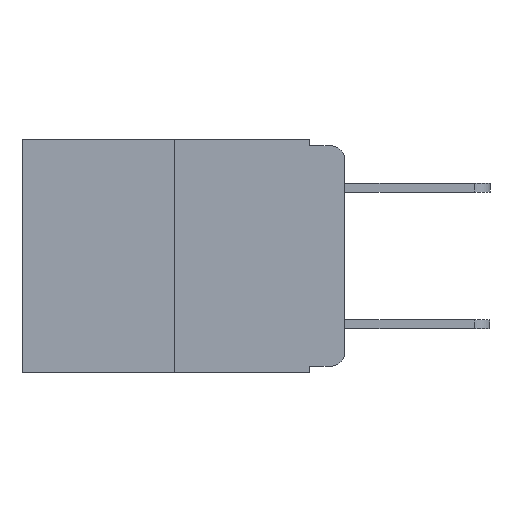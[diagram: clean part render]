
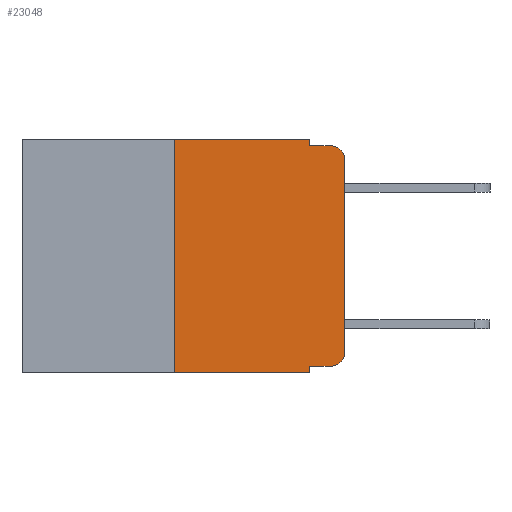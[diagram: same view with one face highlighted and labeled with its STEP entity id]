
A CAD part, left-side view. The second image highlights one B-rep face of the part: STEP entity #23048.
In plain terms, the highlighted planar face has unit normal (-1, 0, 0).
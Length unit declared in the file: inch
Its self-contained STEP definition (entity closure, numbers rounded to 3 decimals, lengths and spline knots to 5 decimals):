
#221 = CARTESIAN_POINT ( 'NONE',  ( 0., 0.02, -0.313 ) ) ;
#282 = CARTESIAN_POINT ( 'NONE',  ( 0., 0.051, -0.01 ) ) ;
#1136 = DIRECTION ( 'NONE',  ( 0., -1., 0. ) ) ;
#1621 = DIRECTION ( 'NONE',  ( 0., 0., -1. ) ) ;
#1648 = VECTOR ( 'NONE', #16089, 39.37008 ) ;
#2386 = DIRECTION ( 'NONE',  ( 0., 0., -1. ) ) ;
#2423 = ORIENTED_EDGE ( 'NONE', *, *, #12696, .T. ) ;
#2565 = LINE ( 'NONE', #9049, #16237 ) ;
#3537 = LINE ( 'NONE', #24974, #13744 ) ;
#3592 = CIRCLE ( 'NONE', #25073, 0.02 ) ;
#4366 = VERTEX_POINT ( 'NONE', #23826 ) ;
#4707 = VERTEX_POINT ( 'NONE', #10649 ) ;
#5667 = LINE ( 'NONE', #11386, #20867 ) ;
#5887 = ORIENTED_EDGE ( 'NONE', *, *, #19730, .T. ) ;
#6065 = CARTESIAN_POINT ( 'NONE',  ( 0., 0.051, 0. ) ) ;
#6078 = EDGE_CURVE ( 'NONE', #4366, #4707, #7816, .T. ) ;
#6690 = ORIENTED_EDGE ( 'NONE', *, *, #21004, .T. ) ;
#6816 = CARTESIAN_POINT ( 'NONE',  ( 0., 0.25, -0.343 ) ) ;
#7063 = DIRECTION ( 'NONE',  ( 0., -1., 0. ) ) ;
#7084 = CARTESIAN_POINT ( 'NONE',  ( 0., 0., -0.03 ) ) ;
#7166 = VECTOR ( 'NONE', #18612, 39.37008 ) ;
#7433 = DIRECTION ( 'NONE',  ( 0., -1., 0. ) ) ;
#7816 = LINE ( 'NONE', #282, #7166 ) ;
#8288 = ORIENTED_EDGE ( 'NONE', *, *, #24489, .T. ) ;
#9049 = CARTESIAN_POINT ( 'NONE',  ( 0., 0.473, -0.343 ) ) ;
#9240 = ORIENTED_EDGE ( 'NONE', *, *, #9906, .F. ) ;
#9301 = ORIENTED_EDGE ( 'NONE', *, *, #25091, .T. ) ;
#9702 = EDGE_CURVE ( 'NONE', #19237, #4366, #18660, .T. ) ;
#9906 = EDGE_CURVE ( 'NONE', #10057, #19237, #3537, .T. ) ;
#10057 = VERTEX_POINT ( 'NONE', #13990 ) ;
#10649 = CARTESIAN_POINT ( 'NONE',  ( 0., 0.02, -0.01 ) ) ;
#10796 = LINE ( 'NONE', #11802, #20591 ) ;
#10855 = CARTESIAN_POINT ( 'NONE',  ( 0., 0.051, 0. ) ) ;
#10887 = VERTEX_POINT ( 'NONE', #7084 ) ;
#10892 = DIRECTION ( 'NONE',  ( 1., 0., 0. ) ) ;
#11386 = CARTESIAN_POINT ( 'NONE',  ( 0., 0.051, -0.333 ) ) ;
#11802 = CARTESIAN_POINT ( 'NONE',  ( 0., 0.25, 0. ) ) ;
#12675 = ORIENTED_EDGE ( 'NONE', *, *, #6078, .F. ) ;
#12696 = EDGE_CURVE ( 'NONE', #20695, #13056, #5667, .T. ) ;
#13056 = VERTEX_POINT ( 'NONE', #14496 ) ;
#13441 = ORIENTED_EDGE ( 'NONE', *, *, #9702, .F. ) ;
#13744 = VECTOR ( 'NONE', #1136, 39.37008 ) ;
#13931 = DIRECTION ( 'NONE',  ( -1., 0., 0. ) ) ;
#13990 = CARTESIAN_POINT ( 'NONE',  ( 0., 0.25, 0. ) ) ;
#14068 = VECTOR ( 'NONE', #24414, 39.37008 ) ;
#14496 = CARTESIAN_POINT ( 'NONE',  ( 0., 0.02, -0.333 ) ) ;
#14610 = DIRECTION ( 'NONE',  ( -1., 0., 0. ) ) ;
#15234 = CARTESIAN_POINT ( 'NONE',  ( 0., 0., -0.313 ) ) ;
#15466 = AXIS2_PLACEMENT_3D ( 'NONE', #25412, #13931, #1621 ) ;
#15663 = FACE_OUTER_BOUND ( 'NONE', #25450, .T. ) ;
#15791 = LINE ( 'NONE', #20997, #24137 ) ;
#16089 = DIRECTION ( 'NONE',  ( 0., 0., -1. ) ) ;
#16237 = VECTOR ( 'NONE', #7063, 39.37008 ) ;
#16926 = CARTESIAN_POINT ( 'NONE',  ( 0., 0.051, 0. ) ) ;
#17564 = CARTESIAN_POINT ( 'NONE',  ( 0., 0.051, -0.333 ) ) ;
#18462 = LINE ( 'NONE', #6065, #1648 ) ;
#18554 = CARTESIAN_POINT ( 'NONE',  ( 0., 0.051, -0.343 ) ) ;
#18612 = DIRECTION ( 'NONE',  ( 0., -1., 0. ) ) ;
#18660 = LINE ( 'NONE', #10855, #14068 ) ;
#19237 = VERTEX_POINT ( 'NONE', #16926 ) ;
#19533 = VERTEX_POINT ( 'NONE', #15234 ) ;
#19730 = EDGE_CURVE ( 'NONE', #10887, #4707, #20257, .T. ) ;
#19788 = EDGE_CURVE ( 'NONE', #20695, #21026, #18462, .T. ) ;
#20257 = CIRCLE ( 'NONE', #15466, 0.02 ) ;
#20591 = VECTOR ( 'NONE', #23388, 39.37008 ) ;
#20645 = PLANE ( 'NONE',  #21790 ) ;
#20695 = VERTEX_POINT ( 'NONE', #17564 ) ;
#20867 = VECTOR ( 'NONE', #7433, 39.37008 ) ;
#20997 = CARTESIAN_POINT ( 'NONE',  ( 0., 0., 0. ) ) ;
#21004 = EDGE_CURVE ( 'NONE', #13056, #19533, #3592, .T. ) ;
#21026 = VERTEX_POINT ( 'NONE', #18554 ) ;
#21087 = VERTEX_POINT ( 'NONE', #6816 ) ;
#21790 = AXIS2_PLACEMENT_3D ( 'NONE', #22442, #10892, #24455 ) ;
#22442 = CARTESIAN_POINT ( 'NONE',  ( 0., 0.473, 0. ) ) ;
#22896 = DIRECTION ( 'NONE',  ( 0., 0., 1. ) ) ;
#23048 = ADVANCED_FACE ( 'NONE', ( #15663 ), #20645, .F. ) ;
#23331 = ORIENTED_EDGE ( 'NONE', *, *, #25277, .F. ) ;
#23388 = DIRECTION ( 'NONE',  ( 0., 0., 1. ) ) ;
#23826 = CARTESIAN_POINT ( 'NONE',  ( 0., 0.051, -0.01 ) ) ;
#24137 = VECTOR ( 'NONE', #22896, 39.37008 ) ;
#24414 = DIRECTION ( 'NONE',  ( 0., 0., -1. ) ) ;
#24455 = DIRECTION ( 'NONE',  ( 0., 0., -1. ) ) ;
#24489 = EDGE_CURVE ( 'NONE', #21087, #21026, #2565, .T. ) ;
#24974 = CARTESIAN_POINT ( 'NONE',  ( 0., 0.473, 0. ) ) ;
#25073 = AXIS2_PLACEMENT_3D ( 'NONE', #221, #14610, #2386 ) ;
#25091 = EDGE_CURVE ( 'NONE', #19533, #10887, #15791, .T. ) ;
#25277 = EDGE_CURVE ( 'NONE', #21087, #10057, #10796, .T. ) ;
#25412 = CARTESIAN_POINT ( 'NONE',  ( 0., 0.02, -0.03 ) ) ;
#25436 = ORIENTED_EDGE ( 'NONE', *, *, #19788, .F. ) ;
#25450 = EDGE_LOOP ( 'NONE', ( #9301, #5887, #12675, #13441, #9240, #23331, #8288, #25436, #2423, #6690 ) ) ;
